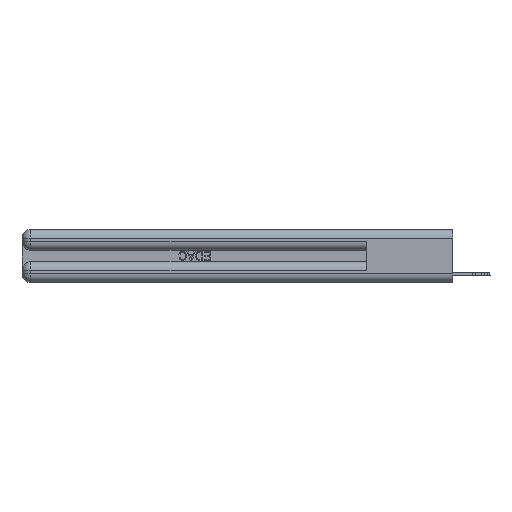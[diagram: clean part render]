
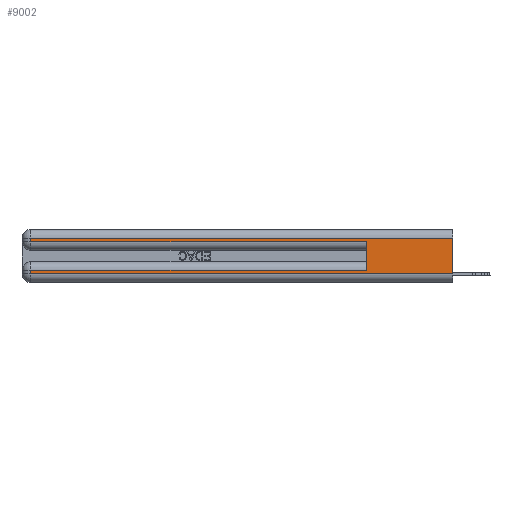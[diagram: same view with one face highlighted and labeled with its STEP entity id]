
A CAD part, left-side view. The second image highlights one B-rep face of the part: STEP entity #9002.
In plain terms, the highlighted planar face has unit normal (-1, 0, 0).
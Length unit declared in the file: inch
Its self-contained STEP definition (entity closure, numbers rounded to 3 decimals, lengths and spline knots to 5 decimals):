
#148 = VECTOR ( 'NONE', #17321, 39.37008 ) ;
#231 = VERTEX_POINT ( 'NONE', #4103 ) ;
#263 = VERTEX_POINT ( 'NONE', #11084 ) ;
#280 = LINE ( 'NONE', #14569, #148 ) ;
#803 = DIRECTION ( 'NONE',  ( 0., 1., 0. ) ) ;
#970 = CARTESIAN_POINT ( 'NONE',  ( 0., 2.94, 0.085 ) ) ;
#2143 = ORIENTED_EDGE ( 'NONE', *, *, #19537, .T. ) ;
#2923 = EDGE_CURVE ( 'NONE', #4258, #231, #27737, .T. ) ;
#2929 = CARTESIAN_POINT ( 'NONE',  ( 0., 0., 0.085 ) ) ;
#3219 = DIRECTION ( 'NONE',  ( 0., 0., -1. ) ) ;
#3225 = CARTESIAN_POINT ( 'NONE',  ( 0., 0., 0.31 ) ) ;
#4103 = CARTESIAN_POINT ( 'NONE',  ( 0., 2.94, 0.06 ) ) ;
#4258 = VERTEX_POINT ( 'NONE', #970 ) ;
#4615 = VERTEX_POINT ( 'NONE', #3225 ) ;
#4646 = VECTOR ( 'NONE', #13453, 39.37008 ) ;
#5156 = CARTESIAN_POINT ( 'NONE',  ( 0., 2.94, 0.37 ) ) ;
#6136 = ORIENTED_EDGE ( 'NONE', *, *, #12794, .T. ) ;
#6916 = LINE ( 'NONE', #29359, #18500 ) ;
#7258 = LINE ( 'NONE', #17178, #18249 ) ;
#7299 = CARTESIAN_POINT ( 'NONE',  ( 0., 2.94, 0.31 ) ) ;
#7759 = FACE_OUTER_BOUND ( 'NONE', #30949, .T. ) ;
#7920 = DIRECTION ( 'NONE',  ( 1., 0., 0. ) ) ;
#8248 = LINE ( 'NONE', #28244, #4646 ) ;
#9002 = ADVANCED_FACE ( 'NONE', ( #7759 ), #15402, .F. ) ;
#9723 = LINE ( 'NONE', #28652, #24560 ) ;
#10014 = DIRECTION ( 'NONE',  ( 0., -1., 0. ) ) ;
#10837 = CARTESIAN_POINT ( 'NONE',  ( 0., 0., 0.37 ) ) ;
#11084 = CARTESIAN_POINT ( 'NONE',  ( 0., 0., 0.06 ) ) ;
#11453 = EDGE_CURVE ( 'NONE', #4615, #263, #8248, .T. ) ;
#12794 = EDGE_CURVE ( 'NONE', #231, #263, #7258, .T. ) ;
#13273 = DIRECTION ( 'NONE',  ( 0., 0., -1. ) ) ;
#13418 = VERTEX_POINT ( 'NONE', #7299 ) ;
#13453 = DIRECTION ( 'NONE',  ( 0., 0., -1. ) ) ;
#13787 = VECTOR ( 'NONE', #26427, 39.37008 ) ;
#14569 = CARTESIAN_POINT ( 'NONE',  ( 0., 0., 0.31 ) ) ;
#14720 = LINE ( 'NONE', #31301, #13787 ) ;
#15316 = VERTEX_POINT ( 'NONE', #31138 ) ;
#15402 = PLANE ( 'NONE',  #23855 ) ;
#15429 = ORIENTED_EDGE ( 'NONE', *, *, #26926, .T. ) ;
#17178 = CARTESIAN_POINT ( 'NONE',  ( 0., 0., 0.06 ) ) ;
#17321 = DIRECTION ( 'NONE',  ( 0., 1., 0. ) ) ;
#18249 = VECTOR ( 'NONE', #10014, 39.37008 ) ;
#18500 = VECTOR ( 'NONE', #19278, 39.37008 ) ;
#19278 = DIRECTION ( 'NONE',  ( 0., 0., 1. ) ) ;
#19283 = CARTESIAN_POINT ( 'NONE',  ( 0., 0.6, 0.285 ) ) ;
#19537 = EDGE_CURVE ( 'NONE', #28025, #4258, #22414, .T. ) ;
#22414 = LINE ( 'NONE', #2929, #23353 ) ;
#22964 = EDGE_CURVE ( 'NONE', #4615, #13418, #280, .T. ) ;
#23054 = ORIENTED_EDGE ( 'NONE', *, *, #11453, .F. ) ;
#23353 = VECTOR ( 'NONE', #803, 39.37008 ) ;
#23764 = DIRECTION ( 'NONE',  ( 0., -1., 0. ) ) ;
#23855 = AXIS2_PLACEMENT_3D ( 'NONE', #10837, #7920, #13273 ) ;
#24513 = ORIENTED_EDGE ( 'NONE', *, *, #22964, .T. ) ;
#24560 = VECTOR ( 'NONE', #23764, 39.37008 ) ;
#24662 = EDGE_CURVE ( 'NONE', #15316, #29929, #9723, .T. ) ;
#25685 = ORIENTED_EDGE ( 'NONE', *, *, #24662, .T. ) ;
#26427 = DIRECTION ( 'NONE',  ( 0., 0., -1. ) ) ;
#26926 = EDGE_CURVE ( 'NONE', #13418, #15316, #14720, .T. ) ;
#27588 = VECTOR ( 'NONE', #3219, 39.37008 ) ;
#27605 = ORIENTED_EDGE ( 'NONE', *, *, #2923, .T. ) ;
#27737 = LINE ( 'NONE', #5156, #27588 ) ;
#28025 = VERTEX_POINT ( 'NONE', #31012 ) ;
#28244 = CARTESIAN_POINT ( 'NONE',  ( 0., 0., 0.37 ) ) ;
#28501 = EDGE_CURVE ( 'NONE', #28025, #29929, #6916, .T. ) ;
#28652 = CARTESIAN_POINT ( 'NONE',  ( 0., 0., 0.285 ) ) ;
#29359 = CARTESIAN_POINT ( 'NONE',  ( 0., 0.6, 0.145 ) ) ;
#29929 = VERTEX_POINT ( 'NONE', #19283 ) ;
#30939 = ORIENTED_EDGE ( 'NONE', *, *, #28501, .F. ) ;
#30949 = EDGE_LOOP ( 'NONE', ( #23054, #24513, #15429, #25685, #30939, #2143, #27605, #6136 ) ) ;
#31012 = CARTESIAN_POINT ( 'NONE',  ( 0., 0.6, 0.085 ) ) ;
#31138 = CARTESIAN_POINT ( 'NONE',  ( 0., 2.94, 0.285 ) ) ;
#31301 = CARTESIAN_POINT ( 'NONE',  ( 0., 2.94, 0.37 ) ) ;
